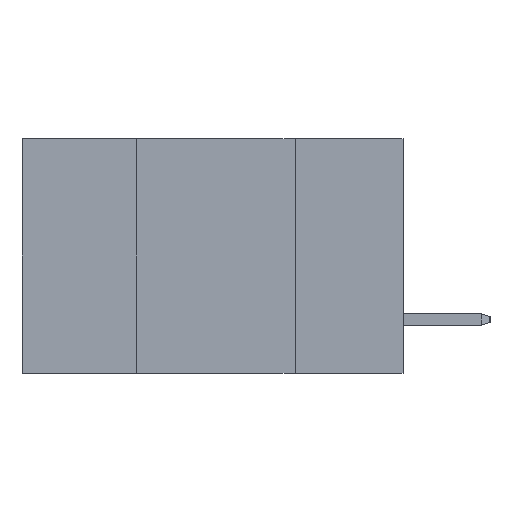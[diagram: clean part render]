
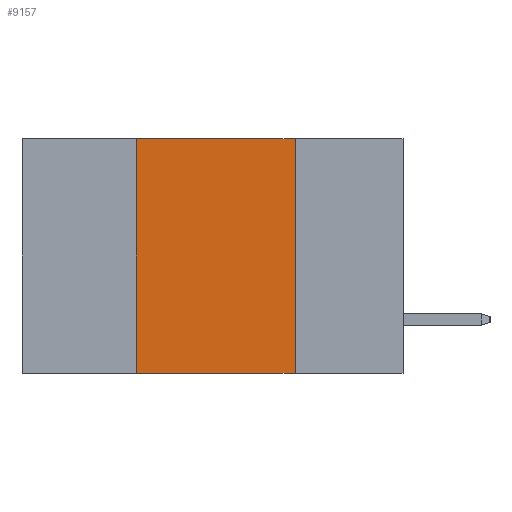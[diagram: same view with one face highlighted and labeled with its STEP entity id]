
A CAD part, left-side view. The second image highlights one B-rep face of the part: STEP entity #9157.
In plain terms, the highlighted planar face has unit normal (-1, 0, 0).
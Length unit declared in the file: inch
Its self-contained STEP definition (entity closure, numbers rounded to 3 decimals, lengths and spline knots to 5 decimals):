
#402 = CARTESIAN_POINT ( 'NONE',  ( 0., 0.42, -0.37 ) ) ;
#678 = EDGE_LOOP ( 'NONE', ( #1300, #5785, #1206, #8760 ) ) ;
#767 = CARTESIAN_POINT ( 'NONE',  ( 0., 0.6, 0. ) ) ;
#1206 = ORIENTED_EDGE ( 'NONE', *, *, #3298, .F. ) ;
#1300 = ORIENTED_EDGE ( 'NONE', *, *, #5171, .F. ) ;
#1388 = VECTOR ( 'NONE', #10085, 39.37008 ) ;
#1564 = DIRECTION ( 'NONE',  ( 0., 0., 1. ) ) ;
#1777 = LINE ( 'NONE', #9461, #5978 ) ;
#1806 = LINE ( 'NONE', #2517, #1388 ) ;
#2229 = EDGE_CURVE ( 'NONE', #3644, #7104, #1777, .T. ) ;
#2517 = CARTESIAN_POINT ( 'NONE',  ( 0., 0.17, 0. ) ) ;
#2656 = CARTESIAN_POINT ( 'NONE',  ( 0., 0.6, -0.37 ) ) ;
#3298 = EDGE_CURVE ( 'NONE', #10543, #3644, #10614, .T. ) ;
#3644 = VERTEX_POINT ( 'NONE', #9414 ) ;
#3909 = DIRECTION ( 'NONE',  ( 0., 0., -1. ) ) ;
#4344 = DIRECTION ( 'NONE',  ( 0., -1., 0. ) ) ;
#4352 = DIRECTION ( 'NONE',  ( 0., -1., 0. ) ) ;
#4567 = AXIS2_PLACEMENT_3D ( 'NONE', #767, #7424, #3909 ) ;
#5171 = EDGE_CURVE ( 'NONE', #7104, #7106, #1806, .T. ) ;
#5785 = ORIENTED_EDGE ( 'NONE', *, *, #2229, .F. ) ;
#5978 = VECTOR ( 'NONE', #4344, 39.37008 ) ;
#6492 = CARTESIAN_POINT ( 'NONE',  ( 0., 0.42, 0. ) ) ;
#7104 = VERTEX_POINT ( 'NONE', #7787 ) ;
#7106 = VERTEX_POINT ( 'NONE', #10350 ) ;
#7424 = DIRECTION ( 'NONE',  ( 1., 0., 0. ) ) ;
#7568 = LINE ( 'NONE', #2656, #10139 ) ;
#7787 = CARTESIAN_POINT ( 'NONE',  ( 0., 0.17, 0. ) ) ;
#8081 = FACE_OUTER_BOUND ( 'NONE', #678, .T. ) ;
#8481 = VECTOR ( 'NONE', #1564, 39.37008 ) ;
#8599 = EDGE_CURVE ( 'NONE', #10543, #7106, #7568, .T. ) ;
#8760 = ORIENTED_EDGE ( 'NONE', *, *, #8599, .T. ) ;
#9157 = ADVANCED_FACE ( 'NONE', ( #8081 ), #9825, .F. ) ;
#9414 = CARTESIAN_POINT ( 'NONE',  ( 0., 0.42, 0. ) ) ;
#9461 = CARTESIAN_POINT ( 'NONE',  ( 0., 0.6, 0. ) ) ;
#9825 = PLANE ( 'NONE',  #4567 ) ;
#10085 = DIRECTION ( 'NONE',  ( 0., 0., -1. ) ) ;
#10139 = VECTOR ( 'NONE', #4352, 39.37008 ) ;
#10350 = CARTESIAN_POINT ( 'NONE',  ( 0., 0.17, -0.37 ) ) ;
#10543 = VERTEX_POINT ( 'NONE', #402 ) ;
#10614 = LINE ( 'NONE', #6492, #8481 ) ;
